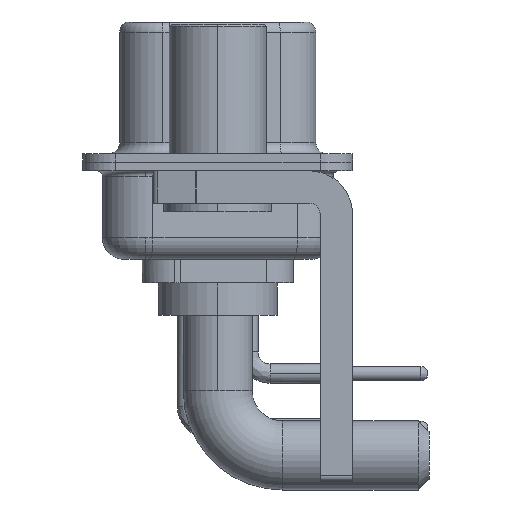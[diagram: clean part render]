
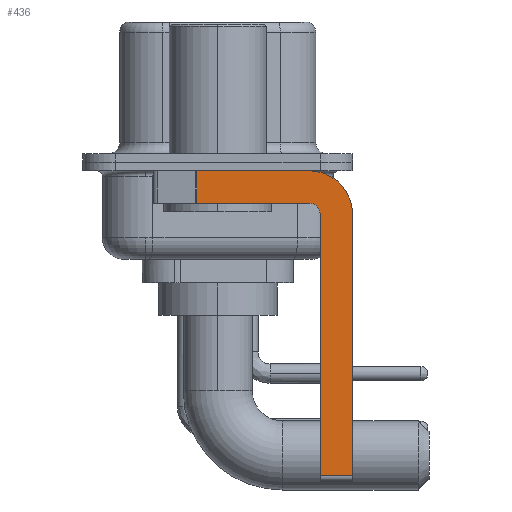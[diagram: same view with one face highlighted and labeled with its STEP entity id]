
A CAD part, left-side view. The second image highlights one B-rep face of the part: STEP entity #436.
In plain terms, the highlighted planar face has unit normal (-1, 0, 0).
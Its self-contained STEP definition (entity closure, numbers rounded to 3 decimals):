
#436 = ADVANCED_FACE ( 'NONE', ( #21732 ), #3610, .F. ) ;
#976 = DIRECTION ( 'NONE',  ( 0., -1., 0. ) ) ;
#1096 = LINE ( 'NONE', #10434, #18343 ) ;
#1244 = VERTEX_POINT ( 'NONE', #23463 ) ;
#1538 = CARTESIAN_POINT ( 'NONE',  ( -2.9, 0.978, -0.4 ) ) ;
#1737 = ORIENTED_EDGE ( 'NONE', *, *, #20019, .F. ) ;
#2764 = CARTESIAN_POINT ( 'NONE',  ( -2.9, -4.25, -14.55 ) ) ;
#2834 = CARTESIAN_POINT ( 'NONE',  ( -2.9, -4.25, -0.4 ) ) ;
#3042 = CIRCLE ( 'NONE', #10955, 0.5 ) ;
#3459 = CARTESIAN_POINT ( 'NONE',  ( -2.9, -6.25, -2.4 ) ) ;
#3610 = PLANE ( 'NONE',  #10364 ) ;
#3897 = CARTESIAN_POINT ( 'NONE',  ( -2.9, 0.978, -1.9 ) ) ;
#4087 = VERTEX_POINT ( 'NONE', #10859 ) ;
#4542 = LINE ( 'NONE', #2764, #22962 ) ;
#5346 = DIRECTION ( 'NONE',  ( 0., 0., -1. ) ) ;
#5815 = EDGE_LOOP ( 'NONE', ( #1737, #9425, #22770, #10118, #8889, #9350, #12408, #17570 ) ) ;
#6908 = VERTEX_POINT ( 'NONE', #1538 ) ;
#6914 = VERTEX_POINT ( 'NONE', #19538 ) ;
#7076 = CARTESIAN_POINT ( 'NONE',  ( -2.9, -4.75, -14.55 ) ) ;
#7753 = LINE ( 'NONE', #11427, #18388 ) ;
#8330 = DIRECTION ( 'NONE',  ( 0., 0., 1. ) ) ;
#8889 = ORIENTED_EDGE ( 'NONE', *, *, #10507, .F. ) ;
#9035 = AXIS2_PLACEMENT_3D ( 'NONE', #18690, #17159, #9671 ) ;
#9207 = CARTESIAN_POINT ( 'NONE',  ( -2.9, -4.75, -2.4 ) ) ;
#9350 = ORIENTED_EDGE ( 'NONE', *, *, #20573, .T. ) ;
#9425 = ORIENTED_EDGE ( 'NONE', *, *, #16949, .T. ) ;
#9671 = DIRECTION ( 'NONE',  ( 0., 0., -1. ) ) ;
#10118 = ORIENTED_EDGE ( 'NONE', *, *, #11376, .F. ) ;
#10364 = AXIS2_PLACEMENT_3D ( 'NONE', #19951, #18190, #10811 ) ;
#10434 = CARTESIAN_POINT ( 'NONE',  ( -2.9, -4.25, -1.9 ) ) ;
#10507 = EDGE_CURVE ( 'NONE', #23234, #19473, #13524, .T. ) ;
#10724 = VECTOR ( 'NONE', #5346, 1000. ) ;
#10811 = DIRECTION ( 'NONE',  ( 0., 0., -1. ) ) ;
#10859 = CARTESIAN_POINT ( 'NONE',  ( -2.9, -4.25, -1.9 ) ) ;
#10955 = AXIS2_PLACEMENT_3D ( 'NONE', #13232, #15156, #13349 ) ;
#11376 = EDGE_CURVE ( 'NONE', #19473, #4087, #3042, .T. ) ;
#11427 = CARTESIAN_POINT ( 'NONE',  ( -2.9, 3., -0.4 ) ) ;
#11469 = VERTEX_POINT ( 'NONE', #2834 ) ;
#12408 = ORIENTED_EDGE ( 'NONE', *, *, #16371, .F. ) ;
#13232 = CARTESIAN_POINT ( 'NONE',  ( -2.9, -4.25, -2.4 ) ) ;
#13349 = DIRECTION ( 'NONE',  ( 0., 0., 1. ) ) ;
#13524 = LINE ( 'NONE', #15586, #18129 ) ;
#14444 = EDGE_CURVE ( 'NONE', #11469, #14501, #19266, .T. ) ;
#14501 = VERTEX_POINT ( 'NONE', #16397 ) ;
#15156 = DIRECTION ( 'NONE',  ( -1., 0., 0. ) ) ;
#15586 = CARTESIAN_POINT ( 'NONE',  ( -2.9, -4.75, -14.8 ) ) ;
#16371 = EDGE_CURVE ( 'NONE', #14501, #6914, #21570, .T. ) ;
#16397 = CARTESIAN_POINT ( 'NONE',  ( -2.9, -6.25, -2.4 ) ) ;
#16949 = EDGE_CURVE ( 'NONE', #6908, #1244, #18809, .T. ) ;
#17159 = DIRECTION ( 'NONE',  ( 1., 0., 0. ) ) ;
#17570 = ORIENTED_EDGE ( 'NONE', *, *, #14444, .F. ) ;
#17679 = EDGE_CURVE ( 'NONE', #4087, #1244, #1096, .T. ) ;
#17682 = DIRECTION ( 'NONE',  ( 0., 1., 0. ) ) ;
#18129 = VECTOR ( 'NONE', #8330, 1000. ) ;
#18190 = DIRECTION ( 'NONE',  ( 1., 0., 0. ) ) ;
#18343 = VECTOR ( 'NONE', #17682, 1000. ) ;
#18388 = VECTOR ( 'NONE', #20444, 1000. ) ;
#18690 = CARTESIAN_POINT ( 'NONE',  ( -2.9, -4.25, -2.4 ) ) ;
#18693 = DIRECTION ( 'NONE',  ( 0., 0., -1. ) ) ;
#18809 = LINE ( 'NONE', #3897, #20220 ) ;
#19266 = CIRCLE ( 'NONE', #9035, 2. ) ;
#19473 = VERTEX_POINT ( 'NONE', #9207 ) ;
#19538 = CARTESIAN_POINT ( 'NONE',  ( -2.9, -6.25, -14.55 ) ) ;
#19951 = CARTESIAN_POINT ( 'NONE',  ( -2.9, -4.25, -2.4 ) ) ;
#20019 = EDGE_CURVE ( 'NONE', #6908, #11469, #7753, .T. ) ;
#20220 = VECTOR ( 'NONE', #18693, 1000. ) ;
#20444 = DIRECTION ( 'NONE',  ( 0., -1., 0. ) ) ;
#20573 = EDGE_CURVE ( 'NONE', #23234, #6914, #4542, .T. ) ;
#21570 = LINE ( 'NONE', #3459, #10724 ) ;
#21732 = FACE_OUTER_BOUND ( 'NONE', #5815, .T. ) ;
#22770 = ORIENTED_EDGE ( 'NONE', *, *, #17679, .F. ) ;
#22962 = VECTOR ( 'NONE', #976, 1000. ) ;
#23234 = VERTEX_POINT ( 'NONE', #7076 ) ;
#23463 = CARTESIAN_POINT ( 'NONE',  ( -2.9, 0.978, -1.9 ) ) ;
